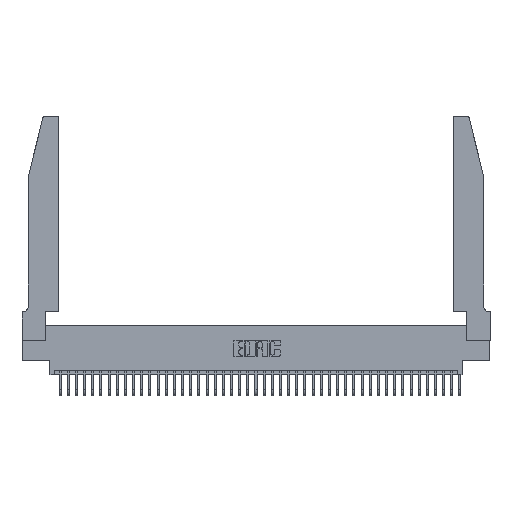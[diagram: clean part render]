
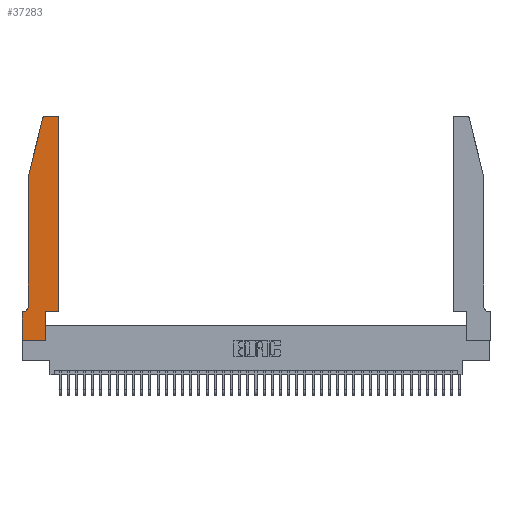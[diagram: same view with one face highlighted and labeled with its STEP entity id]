
A CAD part, top view. The second image highlights one B-rep face of the part: STEP entity #37283.
In plain terms, the highlighted planar face has unit normal (0, 0, 1).
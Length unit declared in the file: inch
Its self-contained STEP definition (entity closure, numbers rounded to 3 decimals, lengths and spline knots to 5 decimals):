
#179 = EDGE_CURVE ( 'NONE', #32085, #574, #3231, .T. ) ;
#574 = VERTEX_POINT ( 'NONE', #31522 ) ;
#1213 = VECTOR ( 'NONE', #32391, 39.37008 ) ;
#1622 = DIRECTION ( 'NONE',  ( 1., 0., 0. ) ) ;
#2318 = CARTESIAN_POINT ( 'NONE',  ( 0.4505, 0.35, 0.37 ) ) ;
#2377 = CARTESIAN_POINT ( 'NONE',  ( 0.0755, 2., 0.37 ) ) ;
#2769 = DIRECTION ( 'NONE',  ( 1., 0., 0. ) ) ;
#3231 = LINE ( 'NONE', #11540, #1213 ) ;
#5248 = PLANE ( 'NONE',  #20708 ) ;
#5603 = CARTESIAN_POINT ( 'NONE',  ( 0.4205, 2.72, 0.37 ) ) ;
#5964 = CARTESIAN_POINT ( 'NONE',  ( 0., 0., 0.37 ) ) ;
#7241 = CARTESIAN_POINT ( 'NONE',  ( 0.0055, 0.42, 0.37 ) ) ;
#7478 = AXIS2_PLACEMENT_3D ( 'NONE', #8035, #30014, #11211 ) ;
#7549 = EDGE_CURVE ( 'NONE', #9621, #37271, #9746, .T. ) ;
#8035 = CARTESIAN_POINT ( 'NONE',  ( 0.284, 2.72, 0.37 ) ) ;
#8489 = DIRECTION ( 'NONE',  ( 0., 0., 1. ) ) ;
#8542 = VERTEX_POINT ( 'NONE', #19772 ) ;
#8719 = ORIENTED_EDGE ( 'NONE', *, *, #11070, .T. ) ;
#8867 = DIRECTION ( 'NONE',  ( 1., 0., 0. ) ) ;
#9008 = VECTOR ( 'NONE', #2769, 39.37008 ) ;
#9078 = DIRECTION ( 'NONE',  ( 0., 1., 0. ) ) ;
#9377 = LINE ( 'NONE', #34235, #16793 ) ;
#9538 = ORIENTED_EDGE ( 'NONE', *, *, #20826, .T. ) ;
#9621 = VERTEX_POINT ( 'NONE', #13409 ) ;
#9746 = CIRCLE ( 'NONE', #29284, 0.03 ) ;
#9869 = CARTESIAN_POINT ( 'NONE',  ( 0.0755, 0.35, 0.37 ) ) ;
#10017 = DIRECTION ( 'NONE',  ( -1., 0., 0. ) ) ;
#10202 = ORIENTED_EDGE ( 'NONE', *, *, #179, .T. ) ;
#10426 = DIRECTION ( 'NONE',  ( -1., 0., 0. ) ) ;
#10636 = VERTEX_POINT ( 'NONE', #39714 ) ;
#10733 = VECTOR ( 'NONE', #1622, 39.37008 ) ;
#10961 = EDGE_LOOP ( 'NONE', ( #39590, #38721, #8719, #10202, #28407, #13251, #23064, #22269, #9538, #16570, #34784, #28836 ) ) ;
#11070 = EDGE_CURVE ( 'NONE', #22875, #32085, #17850, .T. ) ;
#11078 = CARTESIAN_POINT ( 'NONE',  ( 0.0755, 2., 0.37 ) ) ;
#11211 = DIRECTION ( 'NONE',  ( 1., 0., 0. ) ) ;
#11540 = CARTESIAN_POINT ( 'NONE',  ( 0.0755, 2., 0.37 ) ) ;
#11724 = VERTEX_POINT ( 'NONE', #33435 ) ;
#12041 = EDGE_CURVE ( 'NONE', #37271, #28339, #32456, .T. ) ;
#12848 = EDGE_CURVE ( 'NONE', #28339, #22875, #33388, .T. ) ;
#13235 = CARTESIAN_POINT ( 'NONE',  ( 0.2605, 2.75, 0.37 ) ) ;
#13251 = ORIENTED_EDGE ( 'NONE', *, *, #34153, .T. ) ;
#13409 = CARTESIAN_POINT ( 'NONE',  ( 0.4505, 2.72, 0.37 ) ) ;
#13467 = VECTOR ( 'NONE', #29503, 39.37008 ) ;
#14293 = DIRECTION ( 'NONE',  ( -0.239, -0.971, 0. ) ) ;
#14824 = VECTOR ( 'NONE', #10017, 39.37008 ) ;
#15129 = DIRECTION ( 'NONE',  ( 0., -1., 0. ) ) ;
#16141 = VERTEX_POINT ( 'NONE', #28984 ) ;
#16570 = ORIENTED_EDGE ( 'NONE', *, *, #22973, .T. ) ;
#16590 = EDGE_CURVE ( 'NONE', #11724, #16141, #34101, .T. ) ;
#16793 = VECTOR ( 'NONE', #9078, 39.37008 ) ;
#16839 = LINE ( 'NONE', #2318, #40919 ) ;
#17850 = LINE ( 'NONE', #11078, #33536 ) ;
#18106 = DIRECTION ( 'NONE',  ( 0., 1., 0. ) ) ;
#19772 = CARTESIAN_POINT ( 'NONE',  ( 0.0055, 0.35, 0.37 ) ) ;
#20708 = AXIS2_PLACEMENT_3D ( 'NONE', #27263, #8489, #30467 ) ;
#20826 = EDGE_CURVE ( 'NONE', #16141, #29303, #9377, .T. ) ;
#22269 = ORIENTED_EDGE ( 'NONE', *, *, #16590, .T. ) ;
#22875 = VERTEX_POINT ( 'NONE', #28930 ) ;
#22973 = EDGE_CURVE ( 'NONE', #29303, #32736, #35839, .T. ) ;
#23064 = ORIENTED_EDGE ( 'NONE', *, *, #34391, .T. ) ;
#27263 = CARTESIAN_POINT ( 'NONE',  ( 0., 0.35, 0.37 ) ) ;
#27628 = DIRECTION ( 'NONE',  ( 0., 0., 1. ) ) ;
#28339 = VERTEX_POINT ( 'NONE', #36607 ) ;
#28407 = ORIENTED_EDGE ( 'NONE', *, *, #32293, .T. ) ;
#28836 = ORIENTED_EDGE ( 'NONE', *, *, #7549, .T. ) ;
#28930 = CARTESIAN_POINT ( 'NONE',  ( 0.25487, 2.72718, 0.37 ) ) ;
#28984 = CARTESIAN_POINT ( 'NONE',  ( 0.2865, 0., 0.37 ) ) ;
#29223 = DIRECTION ( 'NONE',  ( 0., 0., -1. ) ) ;
#29284 = AXIS2_PLACEMENT_3D ( 'NONE', #5603, #27628, #8867 ) ;
#29303 = VERTEX_POINT ( 'NONE', #38154 ) ;
#29503 = DIRECTION ( 'NONE',  ( -1., 0., 0. ) ) ;
#30014 = DIRECTION ( 'NONE',  ( 0., 0., 1. ) ) ;
#30467 = DIRECTION ( 'NONE',  ( 1., 0., 0. ) ) ;
#30594 = VECTOR ( 'NONE', #15129, 39.37008 ) ;
#30719 = CARTESIAN_POINT ( 'NONE',  ( 0., 0., 0.37 ) ) ;
#31522 = CARTESIAN_POINT ( 'NONE',  ( 0.0755, 0.42, 0.37 ) ) ;
#32085 = VERTEX_POINT ( 'NONE', #2377 ) ;
#32234 = CIRCLE ( 'NONE', #32430, 0.07 ) ;
#32293 = EDGE_CURVE ( 'NONE', #574, #8542, #32234, .T. ) ;
#32391 = DIRECTION ( 'NONE',  ( 0., -1., 0. ) ) ;
#32430 = AXIS2_PLACEMENT_3D ( 'NONE', #7241, #29223, #10426 ) ;
#32456 = LINE ( 'NONE', #13235, #14824 ) ;
#32736 = VERTEX_POINT ( 'NONE', #34474 ) ;
#33388 = CIRCLE ( 'NONE', #7478, 0.03 ) ;
#33435 = CARTESIAN_POINT ( 'NONE',  ( 0., 0., 0.37 ) ) ;
#33536 = VECTOR ( 'NONE', #14293, 39.37008 ) ;
#34101 = LINE ( 'NONE', #5964, #9008 ) ;
#34153 = EDGE_CURVE ( 'NONE', #8542, #10636, #38533, .T. ) ;
#34235 = CARTESIAN_POINT ( 'NONE',  ( 0.2865, 0.35, 0.37 ) ) ;
#34391 = EDGE_CURVE ( 'NONE', #10636, #11724, #39991, .T. ) ;
#34474 = CARTESIAN_POINT ( 'NONE',  ( 0.4505, 0.35, 0.37 ) ) ;
#34784 = ORIENTED_EDGE ( 'NONE', *, *, #39644, .T. ) ;
#35839 = LINE ( 'NONE', #38905, #10733 ) ;
#36607 = CARTESIAN_POINT ( 'NONE',  ( 0.284, 2.75, 0.37 ) ) ;
#37271 = VERTEX_POINT ( 'NONE', #39860 ) ;
#37283 = ADVANCED_FACE ( 'NONE', ( #40806 ), #5248, .T. ) ;
#38154 = CARTESIAN_POINT ( 'NONE',  ( 0.2865, 0.35, 0.37 ) ) ;
#38533 = LINE ( 'NONE', #9869, #13467 ) ;
#38721 = ORIENTED_EDGE ( 'NONE', *, *, #12848, .T. ) ;
#38905 = CARTESIAN_POINT ( 'NONE',  ( 0.4505, 0.35, 0.37 ) ) ;
#39590 = ORIENTED_EDGE ( 'NONE', *, *, #12041, .T. ) ;
#39644 = EDGE_CURVE ( 'NONE', #32736, #9621, #16839, .T. ) ;
#39714 = CARTESIAN_POINT ( 'NONE',  ( 0., 0.35, 0.37 ) ) ;
#39860 = CARTESIAN_POINT ( 'NONE',  ( 0.4205, 2.75, 0.37 ) ) ;
#39991 = LINE ( 'NONE', #30719, #30594 ) ;
#40806 = FACE_OUTER_BOUND ( 'NONE', #10961, .T. ) ;
#40919 = VECTOR ( 'NONE', #18106, 39.37008 ) ;
